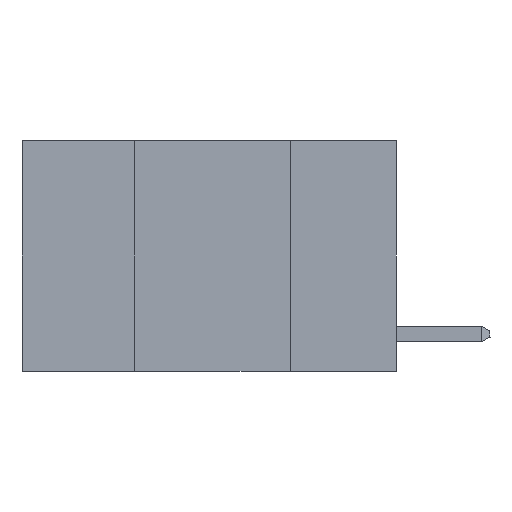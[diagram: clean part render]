
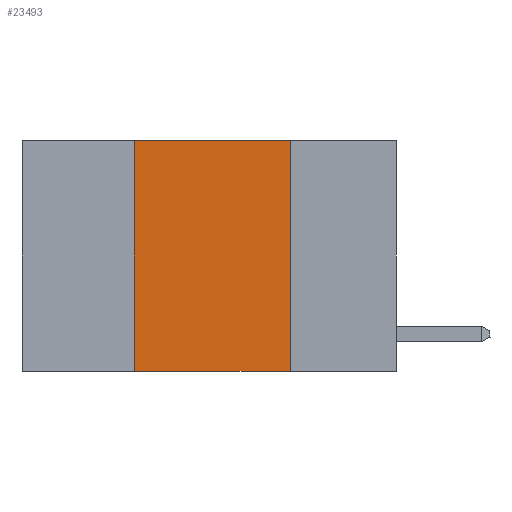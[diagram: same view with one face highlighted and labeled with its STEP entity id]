
A CAD part, left-side view. The second image highlights one B-rep face of the part: STEP entity #23493.
In plain terms, the highlighted planar face has unit normal (-1, 0, 0).
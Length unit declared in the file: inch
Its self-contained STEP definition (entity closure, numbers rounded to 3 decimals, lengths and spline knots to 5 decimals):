
#202 = ORIENTED_EDGE ( 'NONE', *, *, #9848, .F. ) ;
#382 = VECTOR ( 'NONE', #14797, 39.37008 ) ;
#600 = CARTESIAN_POINT ( 'NONE',  ( 0., 0.17, 0. ) ) ;
#725 = VECTOR ( 'NONE', #26147, 39.37008 ) ;
#778 = DIRECTION ( 'NONE',  ( 0., 0., -1. ) ) ;
#1062 = ORIENTED_EDGE ( 'NONE', *, *, #10064, .T. ) ;
#2931 = VERTEX_POINT ( 'NONE', #6389 ) ;
#2952 = LINE ( 'NONE', #7343, #25401 ) ;
#5075 = LINE ( 'NONE', #13695, #11632 ) ;
#5240 = FACE_OUTER_BOUND ( 'NONE', #19708, .T. ) ;
#6389 = CARTESIAN_POINT ( 'NONE',  ( 0., 0.42, -0.37 ) ) ;
#7343 = CARTESIAN_POINT ( 'NONE',  ( 0., 0.17, 0. ) ) ;
#9374 = DIRECTION ( 'NONE',  ( 0., 0., 1. ) ) ;
#9732 = CARTESIAN_POINT ( 'NONE',  ( 0., 0.6, 0. ) ) ;
#9848 = EDGE_CURVE ( 'NONE', #17121, #13371, #12102, .T. ) ;
#10064 = EDGE_CURVE ( 'NONE', #2931, #25555, #23952, .T. ) ;
#11037 = CARTESIAN_POINT ( 'NONE',  ( 0., 0.6, -0.37 ) ) ;
#11632 = VECTOR ( 'NONE', #9374, 39.37008 ) ;
#11933 = DIRECTION ( 'NONE',  ( 0., 0., -1. ) ) ;
#12102 = LINE ( 'NONE', #21159, #382 ) ;
#13371 = VERTEX_POINT ( 'NONE', #600 ) ;
#13695 = CARTESIAN_POINT ( 'NONE',  ( 0., 0.42, 0. ) ) ;
#13980 = EDGE_CURVE ( 'NONE', #13371, #25555, #2952, .T. ) ;
#14797 = DIRECTION ( 'NONE',  ( 0., -1., 0. ) ) ;
#15399 = AXIS2_PLACEMENT_3D ( 'NONE', #9732, #24884, #11933 ) ;
#17121 = VERTEX_POINT ( 'NONE', #17278 ) ;
#17278 = CARTESIAN_POINT ( 'NONE',  ( 0., 0.42, 0. ) ) ;
#17962 = ORIENTED_EDGE ( 'NONE', *, *, #26510, .F. ) ;
#19708 = EDGE_LOOP ( 'NONE', ( #22188, #202, #17962, #1062 ) ) ;
#21069 = CARTESIAN_POINT ( 'NONE',  ( 0., 0.17, -0.37 ) ) ;
#21159 = CARTESIAN_POINT ( 'NONE',  ( 0., 0.6, 0. ) ) ;
#22188 = ORIENTED_EDGE ( 'NONE', *, *, #13980, .F. ) ;
#22747 = PLANE ( 'NONE',  #15399 ) ;
#23493 = ADVANCED_FACE ( 'NONE', ( #5240 ), #22747, .F. ) ;
#23952 = LINE ( 'NONE', #11037, #725 ) ;
#24884 = DIRECTION ( 'NONE',  ( 1., 0., 0. ) ) ;
#25401 = VECTOR ( 'NONE', #778, 39.37008 ) ;
#25555 = VERTEX_POINT ( 'NONE', #21069 ) ;
#26147 = DIRECTION ( 'NONE',  ( 0., -1., 0. ) ) ;
#26510 = EDGE_CURVE ( 'NONE', #2931, #17121, #5075, .T. ) ;
